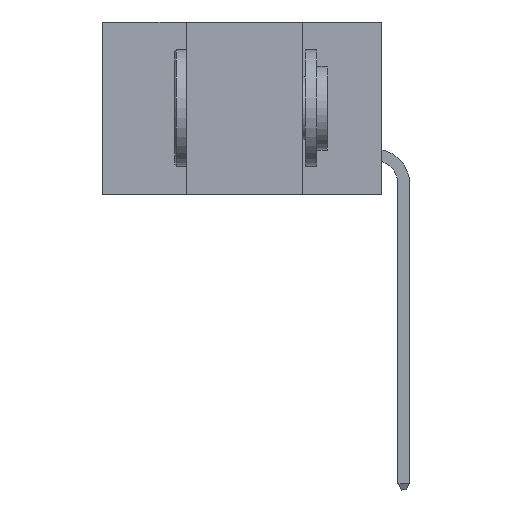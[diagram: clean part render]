
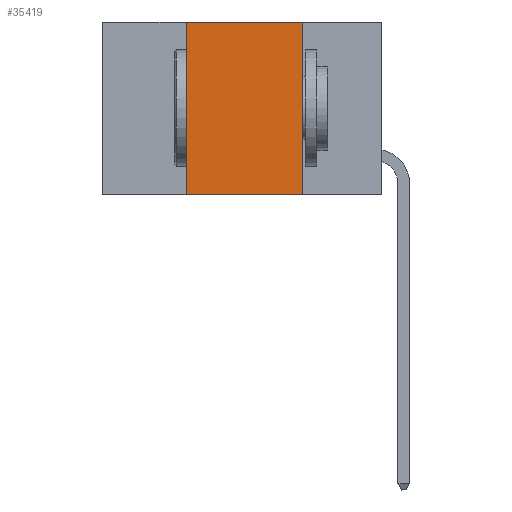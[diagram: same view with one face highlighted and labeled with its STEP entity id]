
A CAD part, left-side view. The second image highlights one B-rep face of the part: STEP entity #35419.
In plain terms, the highlighted planar face has unit normal (-1, 0, 0).
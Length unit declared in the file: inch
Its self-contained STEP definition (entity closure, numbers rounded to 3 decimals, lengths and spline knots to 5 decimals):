
#133 = ORIENTED_EDGE ( 'NONE', *, *, #36742, .F. ) ;
#137 = CARTESIAN_POINT ( 'NONE',  ( 0., 0.17, 0. ) ) ;
#1099 = CARTESIAN_POINT ( 'NONE',  ( 0., 0.6, -0.37 ) ) ;
#1371 = EDGE_LOOP ( 'NONE', ( #47778, #133, #30299, #6640 ) ) ;
#4214 = CARTESIAN_POINT ( 'NONE',  ( 0., 0.6, 0. ) ) ;
#6411 = CARTESIAN_POINT ( 'NONE',  ( 0., 0.42, 0. ) ) ;
#6640 = ORIENTED_EDGE ( 'NONE', *, *, #13596, .T. ) ;
#6800 = CARTESIAN_POINT ( 'NONE',  ( 0., 0.17, 0. ) ) ;
#7641 = AXIS2_PLACEMENT_3D ( 'NONE', #36372, #21250, #40041 ) ;
#10474 = DIRECTION ( 'NONE',  ( 0., -1., 0. ) ) ;
#12738 = EDGE_CURVE ( 'NONE', #43455, #28106, #13038, .T. ) ;
#13038 = LINE ( 'NONE', #6800, #38619 ) ;
#13596 = EDGE_CURVE ( 'NONE', #15267, #28106, #17026, .T. ) ;
#13914 = PLANE ( 'NONE',  #7641 ) ;
#14761 = VECTOR ( 'NONE', #34506, 39.37008 ) ;
#15267 = VERTEX_POINT ( 'NONE', #16357 ) ;
#16357 = CARTESIAN_POINT ( 'NONE',  ( 0., 0.42, -0.37 ) ) ;
#16488 = CARTESIAN_POINT ( 'NONE',  ( 0., 0.17, -0.37 ) ) ;
#17026 = LINE ( 'NONE', #1099, #27495 ) ;
#19831 = FACE_OUTER_BOUND ( 'NONE', #1371, .T. ) ;
#21250 = DIRECTION ( 'NONE',  ( 1., 0., 0. ) ) ;
#26546 = CARTESIAN_POINT ( 'NONE',  ( 0., 0.42, 0. ) ) ;
#27495 = VECTOR ( 'NONE', #10474, 39.37008 ) ;
#28106 = VERTEX_POINT ( 'NONE', #16488 ) ;
#30299 = ORIENTED_EDGE ( 'NONE', *, *, #33890, .F. ) ;
#30784 = VERTEX_POINT ( 'NONE', #6411 ) ;
#33389 = LINE ( 'NONE', #26546, #14761 ) ;
#33890 = EDGE_CURVE ( 'NONE', #15267, #30784, #33389, .T. ) ;
#34506 = DIRECTION ( 'NONE',  ( 0., 0., 1. ) ) ;
#34875 = LINE ( 'NONE', #4214, #35505 ) ;
#35419 = ADVANCED_FACE ( 'NONE', ( #19831 ), #13914, .F. ) ;
#35505 = VECTOR ( 'NONE', #44534, 39.37008 ) ;
#36372 = CARTESIAN_POINT ( 'NONE',  ( 0., 0.6, 0. ) ) ;
#36742 = EDGE_CURVE ( 'NONE', #30784, #43455, #34875, .T. ) ;
#38619 = VECTOR ( 'NONE', #47715, 39.37008 ) ;
#40041 = DIRECTION ( 'NONE',  ( 0., 0., -1. ) ) ;
#43455 = VERTEX_POINT ( 'NONE', #137 ) ;
#44534 = DIRECTION ( 'NONE',  ( 0., -1., 0. ) ) ;
#47715 = DIRECTION ( 'NONE',  ( 0., 0., -1. ) ) ;
#47778 = ORIENTED_EDGE ( 'NONE', *, *, #12738, .F. ) ;
